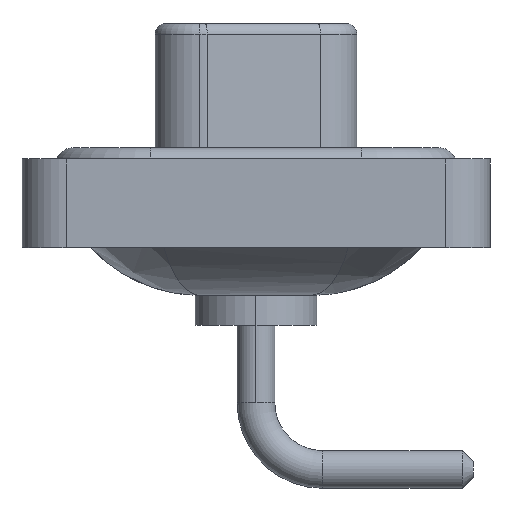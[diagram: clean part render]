
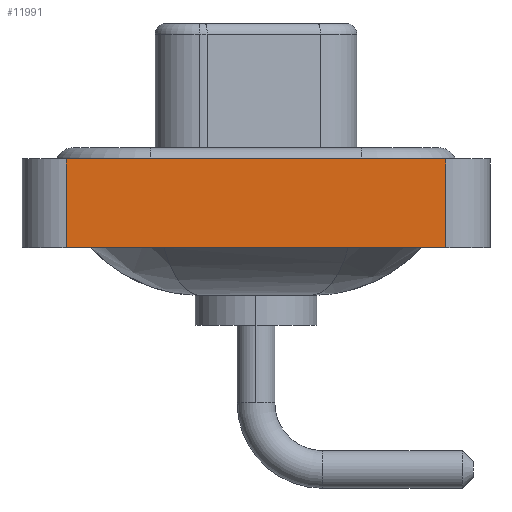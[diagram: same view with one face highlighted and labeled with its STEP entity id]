
A CAD part, left-side view. The second image highlights one B-rep face of the part: STEP entity #11991.
In plain terms, the highlighted planar face has unit normal (-1, 0, 0).
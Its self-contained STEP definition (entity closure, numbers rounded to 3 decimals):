
#133 = DIRECTION ( 'NONE',  ( 0., 0., 1. ) ) ;
#324 = VECTOR ( 'NONE', #621, 1000. ) ;
#438 = CARTESIAN_POINT ( 'NONE',  ( -7.25, -8.55, -3.6 ) ) ;
#475 = VECTOR ( 'NONE', #133, 1000. ) ;
#621 = DIRECTION ( 'NONE',  ( 0., -1., 0. ) ) ;
#712 = VERTEX_POINT ( 'NONE', #4689 ) ;
#763 = CARTESIAN_POINT ( 'NONE',  ( -7.25, -8.55, -3.6 ) ) ;
#1253 = EDGE_LOOP ( 'NONE', ( #3551, #9411, #3972, #14361 ) ) ;
#2196 = LINE ( 'NONE', #5960, #475 ) ;
#2235 = PLANE ( 'NONE',  #4829 ) ;
#2608 = VECTOR ( 'NONE', #5123, 1000. ) ;
#3148 = FACE_OUTER_BOUND ( 'NONE', #1253, .T. ) ;
#3551 = ORIENTED_EDGE ( 'NONE', *, *, #4260, .T. ) ;
#3972 = ORIENTED_EDGE ( 'NONE', *, *, #14222, .F. ) ;
#4013 = LINE ( 'NONE', #7451, #5544 ) ;
#4260 = EDGE_CURVE ( 'NONE', #6791, #8473, #13238, .T. ) ;
#4458 = CARTESIAN_POINT ( 'NONE',  ( -7.25, -8.55, -3.6 ) ) ;
#4689 = CARTESIAN_POINT ( 'NONE',  ( -7.25, 8.55, 0.4 ) ) ;
#4829 = AXIS2_PLACEMENT_3D ( 'NONE', #4458, #10174, #12428 ) ;
#5123 = DIRECTION ( 'NONE',  ( 0., 0., 1. ) ) ;
#5544 = VECTOR ( 'NONE', #12279, 1000. ) ;
#5960 = CARTESIAN_POINT ( 'NONE',  ( -7.25, 8.55, -3.6 ) ) ;
#6104 = CARTESIAN_POINT ( 'NONE',  ( -7.25, -8.55, -3.6 ) ) ;
#6791 = VERTEX_POINT ( 'NONE', #6104 ) ;
#6876 = EDGE_CURVE ( 'NONE', #12522, #6791, #11266, .T. ) ;
#7386 = CARTESIAN_POINT ( 'NONE',  ( -7.25, -8.55, 0.4 ) ) ;
#7451 = CARTESIAN_POINT ( 'NONE',  ( -7.25, -8.55, 0.4 ) ) ;
#8473 = VERTEX_POINT ( 'NONE', #7386 ) ;
#9411 = ORIENTED_EDGE ( 'NONE', *, *, #11885, .F. ) ;
#9416 = CARTESIAN_POINT ( 'NONE',  ( -7.25, 8.55, -3.6 ) ) ;
#10174 = DIRECTION ( 'NONE',  ( -1., 0., 0. ) ) ;
#11266 = LINE ( 'NONE', #763, #324 ) ;
#11885 = EDGE_CURVE ( 'NONE', #712, #8473, #4013, .T. ) ;
#11991 = ADVANCED_FACE ( 'NONE', ( #3148 ), #2235, .T. ) ;
#12279 = DIRECTION ( 'NONE',  ( 0., -1., 0. ) ) ;
#12428 = DIRECTION ( 'NONE',  ( 0., 0., 1. ) ) ;
#12522 = VERTEX_POINT ( 'NONE', #9416 ) ;
#13238 = LINE ( 'NONE', #438, #2608 ) ;
#14222 = EDGE_CURVE ( 'NONE', #12522, #712, #2196, .T. ) ;
#14361 = ORIENTED_EDGE ( 'NONE', *, *, #6876, .T. ) ;
